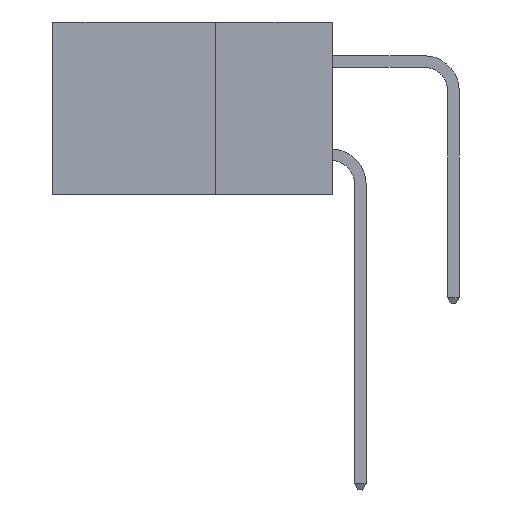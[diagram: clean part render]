
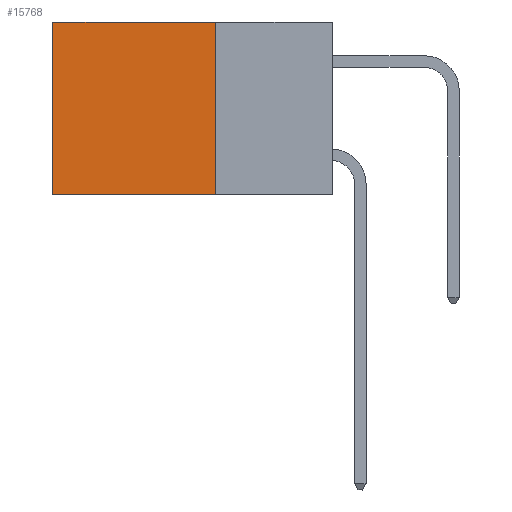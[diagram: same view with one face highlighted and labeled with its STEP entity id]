
A CAD part, left-side view. The second image highlights one B-rep face of the part: STEP entity #15768.
In plain terms, the highlighted planar face has unit normal (-1, 0, 0).
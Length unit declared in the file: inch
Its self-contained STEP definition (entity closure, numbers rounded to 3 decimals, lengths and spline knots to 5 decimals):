
#363 = ORIENTED_EDGE ( 'NONE', *, *, #2774, .F. ) ;
#996 = DIRECTION ( 'NONE',  ( 0., 0., -1. ) ) ;
#1090 = VERTEX_POINT ( 'NONE', #19283 ) ;
#1388 = VECTOR ( 'NONE', #9372, 39.37008 ) ;
#2014 = VERTEX_POINT ( 'NONE', #19788 ) ;
#2300 = DIRECTION ( 'NONE',  ( 0., 0., -1. ) ) ;
#2302 = EDGE_CURVE ( 'NONE', #15713, #2014, #11195, .T. ) ;
#2774 = EDGE_CURVE ( 'NONE', #1090, #15427, #16943, .T. ) ;
#3593 = EDGE_LOOP ( 'NONE', ( #12745, #10849, #363, #8458 ) ) ;
#3703 = EDGE_CURVE ( 'NONE', #1090, #15713, #4549, .T. ) ;
#4492 = CARTESIAN_POINT ( 'NONE',  ( 0.298, 0.6, 0. ) ) ;
#4549 = LINE ( 'NONE', #8663, #16429 ) ;
#4600 = CARTESIAN_POINT ( 'NONE',  ( 0.298, 0.25, -0.37 ) ) ;
#5210 = CARTESIAN_POINT ( 'NONE',  ( 0.298, 0.6, 0. ) ) ;
#5404 = EDGE_CURVE ( 'NONE', #15427, #2014, #8998, .T. ) ;
#7710 = DIRECTION ( 'NONE',  ( 0., 1., 0. ) ) ;
#8458 = ORIENTED_EDGE ( 'NONE', *, *, #3703, .T. ) ;
#8663 = CARTESIAN_POINT ( 'NONE',  ( 0.298, 0.25, 0. ) ) ;
#8998 = LINE ( 'NONE', #4600, #13287 ) ;
#9372 = DIRECTION ( 'NONE',  ( 0., 0., -1. ) ) ;
#9978 = CARTESIAN_POINT ( 'NONE',  ( 0.298, 0.25, 0. ) ) ;
#10673 = VECTOR ( 'NONE', #996, 39.37008 ) ;
#10731 = CARTESIAN_POINT ( 'NONE',  ( 0.298, 0.25, -0.37 ) ) ;
#10849 = ORIENTED_EDGE ( 'NONE', *, *, #5404, .F. ) ;
#11195 = LINE ( 'NONE', #4492, #10673 ) ;
#11641 = DIRECTION ( 'NONE',  ( 1., 0., 0. ) ) ;
#12745 = ORIENTED_EDGE ( 'NONE', *, *, #2302, .T. ) ;
#13287 = VECTOR ( 'NONE', #7710, 39.37008 ) ;
#14085 = CARTESIAN_POINT ( 'NONE',  ( 0.298, 0.25, 0. ) ) ;
#15427 = VERTEX_POINT ( 'NONE', #10731 ) ;
#15517 = FACE_OUTER_BOUND ( 'NONE', #3593, .T. ) ;
#15713 = VERTEX_POINT ( 'NONE', #5210 ) ;
#15768 = ADVANCED_FACE ( 'NONE', ( #15517 ), #19212, .F. ) ;
#15844 = DIRECTION ( 'NONE',  ( 0., 1., 0. ) ) ;
#16429 = VECTOR ( 'NONE', #15844, 39.37008 ) ;
#16943 = LINE ( 'NONE', #14085, #1388 ) ;
#19212 = PLANE ( 'NONE',  #19309 ) ;
#19283 = CARTESIAN_POINT ( 'NONE',  ( 0.298, 0.25, 0. ) ) ;
#19309 = AXIS2_PLACEMENT_3D ( 'NONE', #9978, #11641, #2300 ) ;
#19788 = CARTESIAN_POINT ( 'NONE',  ( 0.298, 0.6, -0.37 ) ) ;
